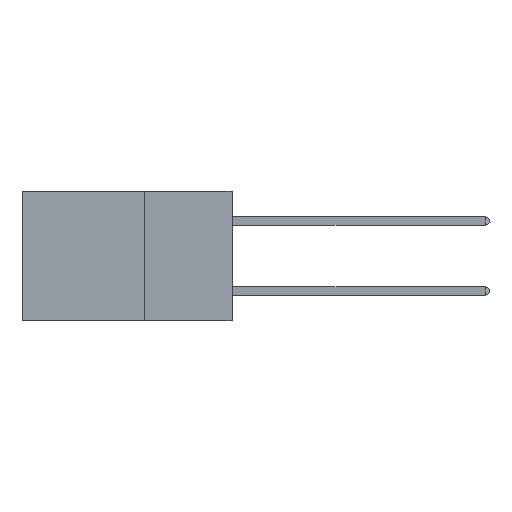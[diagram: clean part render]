
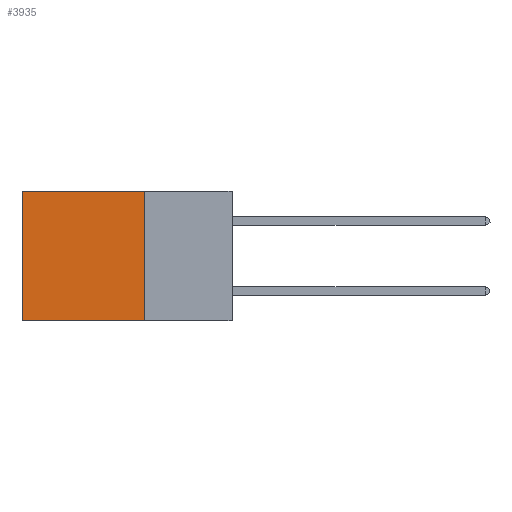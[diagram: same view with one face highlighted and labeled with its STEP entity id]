
A CAD part, left-side view. The second image highlights one B-rep face of the part: STEP entity #3935.
In plain terms, the highlighted planar face has unit normal (-1, 0, 0).
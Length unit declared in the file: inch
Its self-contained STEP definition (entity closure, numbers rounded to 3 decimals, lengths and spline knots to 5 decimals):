
#50 = ORIENTED_EDGE ( 'NONE', *, *, #6734, .T. ) ;
#208 = DIRECTION ( 'NONE',  ( 0., 0., -1. ) ) ;
#390 = VECTOR ( 'NONE', #6129, 39.37008 ) ;
#1408 = DIRECTION ( 'NONE',  ( 1., 0., 0. ) ) ;
#1486 = CARTESIAN_POINT ( 'NONE',  ( 0.2875, 0.25, 0. ) ) ;
#1820 = LINE ( 'NONE', #10215, #4269 ) ;
#2824 = ORIENTED_EDGE ( 'NONE', *, *, #3737, .T. ) ;
#3314 = DIRECTION ( 'NONE',  ( 0., 0., -1. ) ) ;
#3537 = ORIENTED_EDGE ( 'NONE', *, *, #14189, .F. ) ;
#3737 = EDGE_CURVE ( 'NONE', #8928, #6642, #3993, .T. ) ;
#3935 = ADVANCED_FACE ( 'NONE', ( #13444 ), #4112, .F. ) ;
#3993 = LINE ( 'NONE', #7634, #10043 ) ;
#4112 = PLANE ( 'NONE',  #13818 ) ;
#4269 = VECTOR ( 'NONE', #11469, 39.37008 ) ;
#4781 = EDGE_CURVE ( 'NONE', #7937, #7377, #7555, .T. ) ;
#5027 = CARTESIAN_POINT ( 'NONE',  ( 0.2875, 0.6, -0.37 ) ) ;
#6129 = DIRECTION ( 'NONE',  ( 0., 1., 0. ) ) ;
#6562 = CARTESIAN_POINT ( 'NONE',  ( 0.2875, 0.6, 0. ) ) ;
#6642 = VERTEX_POINT ( 'NONE', #6562 ) ;
#6734 = EDGE_CURVE ( 'NONE', #6642, #7377, #10510, .T. ) ;
#7377 = VERTEX_POINT ( 'NONE', #5027 ) ;
#7555 = LINE ( 'NONE', #9854, #390 ) ;
#7634 = CARTESIAN_POINT ( 'NONE',  ( 0.2875, 0.25, 0. ) ) ;
#7937 = VERTEX_POINT ( 'NONE', #9194 ) ;
#8827 = VECTOR ( 'NONE', #3314, 39.37008 ) ;
#8928 = VERTEX_POINT ( 'NONE', #15381 ) ;
#9194 = CARTESIAN_POINT ( 'NONE',  ( 0.2875, 0.25, -0.37 ) ) ;
#9854 = CARTESIAN_POINT ( 'NONE',  ( 0.2875, 0.25, -0.37 ) ) ;
#10009 = ORIENTED_EDGE ( 'NONE', *, *, #4781, .F. ) ;
#10043 = VECTOR ( 'NONE', #12447, 39.37008 ) ;
#10215 = CARTESIAN_POINT ( 'NONE',  ( 0.2875, 0.25, 0. ) ) ;
#10510 = LINE ( 'NONE', #15337, #8827 ) ;
#11469 = DIRECTION ( 'NONE',  ( 0., 0., -1. ) ) ;
#12447 = DIRECTION ( 'NONE',  ( 0., 1., 0. ) ) ;
#13444 = FACE_OUTER_BOUND ( 'NONE', #15294, .T. ) ;
#13818 = AXIS2_PLACEMENT_3D ( 'NONE', #1486, #1408, #208 ) ;
#14189 = EDGE_CURVE ( 'NONE', #8928, #7937, #1820, .T. ) ;
#15294 = EDGE_LOOP ( 'NONE', ( #50, #10009, #3537, #2824 ) ) ;
#15337 = CARTESIAN_POINT ( 'NONE',  ( 0.2875, 0.6, 0. ) ) ;
#15381 = CARTESIAN_POINT ( 'NONE',  ( 0.2875, 0.25, 0. ) ) ;
